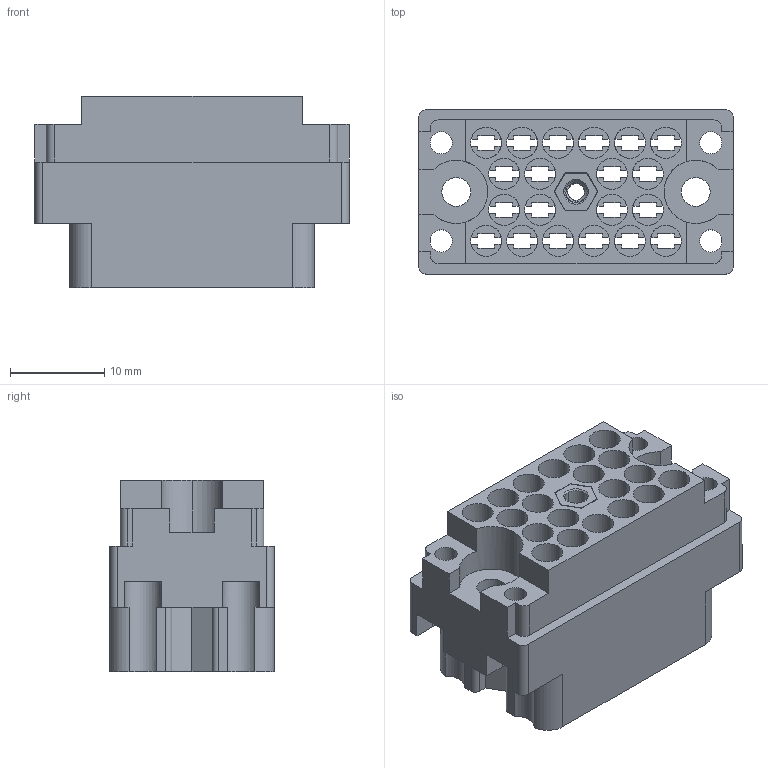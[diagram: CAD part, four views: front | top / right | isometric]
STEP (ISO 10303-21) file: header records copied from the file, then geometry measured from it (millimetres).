
FILE_DESCRIPTION (( 'STEP AP203' ), '1' );
FILE_NAME ('516-020-000-506.STEP', '2020-03-09T13:04:18', ( '' ), ( '' ), 'SwSTEP 2.0', 'SolidWorks 2016', '' );
FILE_SCHEMA (( 'CONFIG_CONTROL_DESIGN' ));
Length unit declared in the file: inch
Products named in the file (3): 516 Plug Insulator_020; 516-020-000-506; 516-252-025-100_516-252-025-100
Assembly tree (2 placements, depth 2):
  516-020-000-506
    516 Plug Insulator_020
    516-252-025-100_516-252-025-100
Bounding box: 33.32 x 17.42 x 20.27 mm (x, y, z)
Volume: 4453.5 mm3; surface area: 7229.2 mm2
Topology: 2 solids, 2 shells, 666 faces, 1940 edges, 1289 vertices
Faces by surface type: plane 442, cylinder 210, cone 11, bspline 3
Entity records: 24965 total; most frequent: CARTESIAN_POINT 6616, ORIENTED_EDGE 3880, DIRECTION 3695, EDGE_CURVE 1940, LINE 1409, VECTOR 1409, VERTEX_POINT 1289, AXIS2_PLACEMENT_3D 1143
